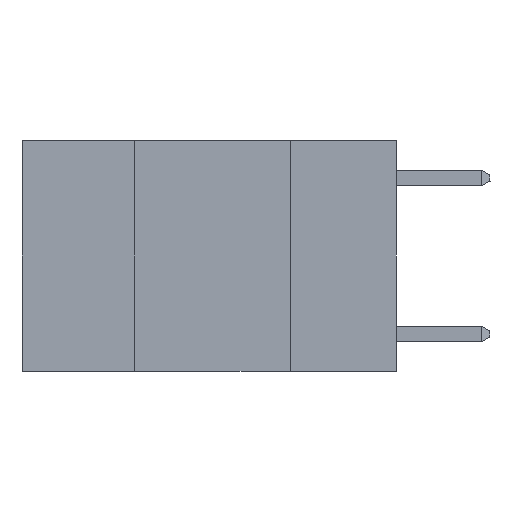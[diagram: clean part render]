
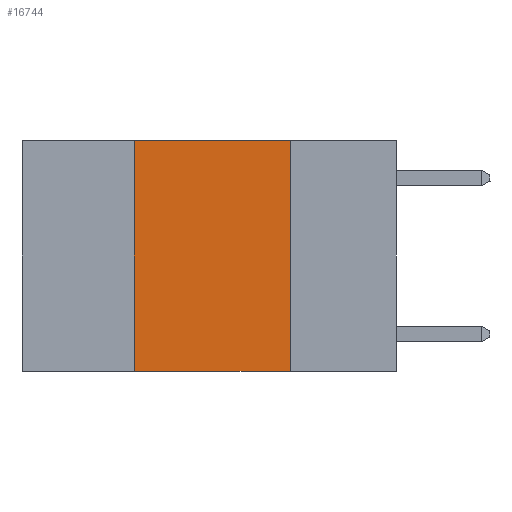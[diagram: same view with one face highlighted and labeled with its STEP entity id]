
A CAD part, left-side view. The second image highlights one B-rep face of the part: STEP entity #16744.
In plain terms, the highlighted planar face has unit normal (-1, 0, 0).
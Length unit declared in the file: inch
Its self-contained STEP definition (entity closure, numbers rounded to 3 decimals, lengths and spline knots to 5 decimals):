
#2467 = ORIENTED_EDGE ( 'NONE', *, *, #22854, .T. ) ;
#3010 = VERTEX_POINT ( 'NONE', #7593 ) ;
#3011 = CARTESIAN_POINT ( 'NONE',  ( 0., 0.6, -0.37 ) ) ;
#3055 = ORIENTED_EDGE ( 'NONE', *, *, #4113, .F. ) ;
#3338 = DIRECTION ( 'NONE',  ( 0., 0., 1. ) ) ;
#4113 = EDGE_CURVE ( 'NONE', #20572, #3010, #12241, .T. ) ;
#7021 = CARTESIAN_POINT ( 'NONE',  ( 0., 0.17, 0. ) ) ;
#7460 = DIRECTION ( 'NONE',  ( 1., 0., 0. ) ) ;
#7593 = CARTESIAN_POINT ( 'NONE',  ( 0., 0.17, 0. ) ) ;
#8119 = VERTEX_POINT ( 'NONE', #14628 ) ;
#8417 = EDGE_CURVE ( 'NONE', #8119, #20572, #26735, .T. ) ;
#9583 = VECTOR ( 'NONE', #3338, 39.37008 ) ;
#10459 = VECTOR ( 'NONE', #16413, 39.37008 ) ;
#11756 = VECTOR ( 'NONE', #13573, 39.37008 ) ;
#12241 = LINE ( 'NONE', #22976, #10459 ) ;
#12623 = ORIENTED_EDGE ( 'NONE', *, *, #8417, .F. ) ;
#13573 = DIRECTION ( 'NONE',  ( 0., 0., -1. ) ) ;
#14628 = CARTESIAN_POINT ( 'NONE',  ( 0., 0.42, -0.37 ) ) ;
#15389 = LINE ( 'NONE', #7021, #11756 ) ;
#16142 = CARTESIAN_POINT ( 'NONE',  ( 0., 0.42, 0. ) ) ;
#16413 = DIRECTION ( 'NONE',  ( 0., -1., 0. ) ) ;
#16744 = ADVANCED_FACE ( 'NONE', ( #24891 ), #22527, .F. ) ;
#16813 = ORIENTED_EDGE ( 'NONE', *, *, #18368, .F. ) ;
#18368 = EDGE_CURVE ( 'NONE', #3010, #26761, #15389, .T. ) ;
#19119 = CARTESIAN_POINT ( 'NONE',  ( 0., 0.6, 0. ) ) ;
#19773 = AXIS2_PLACEMENT_3D ( 'NONE', #19119, #7460, #24765 ) ;
#19856 = DIRECTION ( 'NONE',  ( 0., -1., 0. ) ) ;
#19897 = CARTESIAN_POINT ( 'NONE',  ( 0., 0.17, -0.37 ) ) ;
#20572 = VERTEX_POINT ( 'NONE', #27150 ) ;
#22527 = PLANE ( 'NONE',  #19773 ) ;
#22613 = EDGE_LOOP ( 'NONE', ( #16813, #3055, #12623, #2467 ) ) ;
#22854 = EDGE_CURVE ( 'NONE', #8119, #26761, #24191, .T. ) ;
#22976 = CARTESIAN_POINT ( 'NONE',  ( 0., 0.6, 0. ) ) ;
#24191 = LINE ( 'NONE', #3011, #25414 ) ;
#24765 = DIRECTION ( 'NONE',  ( 0., 0., -1. ) ) ;
#24891 = FACE_OUTER_BOUND ( 'NONE', #22613, .T. ) ;
#25414 = VECTOR ( 'NONE', #19856, 39.37008 ) ;
#26735 = LINE ( 'NONE', #16142, #9583 ) ;
#26761 = VERTEX_POINT ( 'NONE', #19897 ) ;
#27150 = CARTESIAN_POINT ( 'NONE',  ( 0., 0.42, 0. ) ) ;
